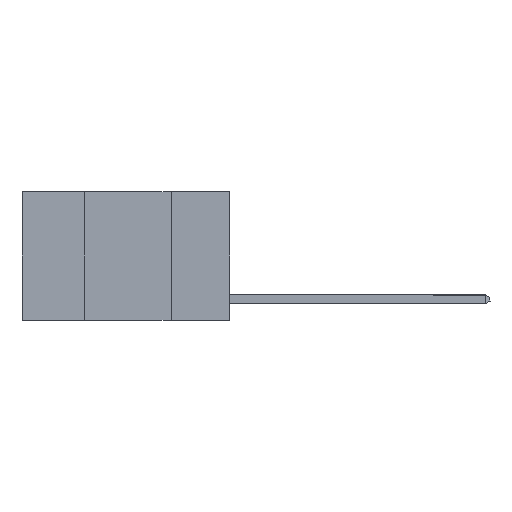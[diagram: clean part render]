
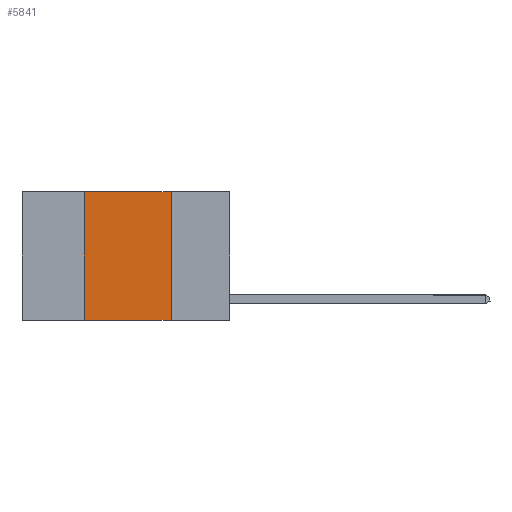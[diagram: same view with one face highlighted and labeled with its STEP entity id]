
A CAD part, left-side view. The second image highlights one B-rep face of the part: STEP entity #5841.
In plain terms, the highlighted planar face has unit normal (-1, 0, 0).
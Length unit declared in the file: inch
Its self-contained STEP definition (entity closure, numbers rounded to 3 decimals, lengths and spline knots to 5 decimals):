
#486 = LINE ( 'NONE', #6001, #4030 ) ;
#499 = EDGE_CURVE ( 'NONE', #4530, #4029, #4433, .T. ) ;
#816 = CARTESIAN_POINT ( 'NONE',  ( 0., 0.42, 0. ) ) ;
#873 = LINE ( 'NONE', #2866, #8140 ) ;
#902 = DIRECTION ( 'NONE',  ( 1., 0., 0. ) ) ;
#1607 = DIRECTION ( 'NONE',  ( 0., -1., 0. ) ) ;
#2190 = LINE ( 'NONE', #3654, #5828 ) ;
#2866 = CARTESIAN_POINT ( 'NONE',  ( 0., 0.42, 0. ) ) ;
#2947 = EDGE_CURVE ( 'NONE', #5457, #4029, #2190, .T. ) ;
#3586 = DIRECTION ( 'NONE',  ( 0., 0., 1. ) ) ;
#3654 = CARTESIAN_POINT ( 'NONE',  ( 0., 0.6, -0.37 ) ) ;
#3820 = CARTESIAN_POINT ( 'NONE',  ( 0., 0.17, 0. ) ) ;
#3882 = PLANE ( 'NONE',  #5989 ) ;
#4029 = VERTEX_POINT ( 'NONE', #6752 ) ;
#4030 = VECTOR ( 'NONE', #1607, 39.37008 ) ;
#4433 = LINE ( 'NONE', #3820, #8183 ) ;
#4530 = VERTEX_POINT ( 'NONE', #8674 ) ;
#4539 = DIRECTION ( 'NONE',  ( 0., 0., -1. ) ) ;
#4798 = CARTESIAN_POINT ( 'NONE',  ( 0., 0.42, -0.37 ) ) ;
#4890 = ORIENTED_EDGE ( 'NONE', *, *, #499, .F. ) ;
#5123 = ORIENTED_EDGE ( 'NONE', *, *, #6675, .F. ) ;
#5340 = CARTESIAN_POINT ( 'NONE',  ( 0., 0.6, 0. ) ) ;
#5457 = VERTEX_POINT ( 'NONE', #4798 ) ;
#5828 = VECTOR ( 'NONE', #7919, 39.37008 ) ;
#5841 = ADVANCED_FACE ( 'NONE', ( #7607 ), #3882, .F. ) ;
#5989 = AXIS2_PLACEMENT_3D ( 'NONE', #5340, #902, #6048 ) ;
#6001 = CARTESIAN_POINT ( 'NONE',  ( 0., 0.6, 0. ) ) ;
#6048 = DIRECTION ( 'NONE',  ( 0., 0., -1. ) ) ;
#6413 = EDGE_CURVE ( 'NONE', #5457, #8448, #873, .T. ) ;
#6675 = EDGE_CURVE ( 'NONE', #8448, #4530, #486, .T. ) ;
#6752 = CARTESIAN_POINT ( 'NONE',  ( 0., 0.17, -0.37 ) ) ;
#6988 = ORIENTED_EDGE ( 'NONE', *, *, #6413, .F. ) ;
#7607 = FACE_OUTER_BOUND ( 'NONE', #8508, .T. ) ;
#7919 = DIRECTION ( 'NONE',  ( 0., -1., 0. ) ) ;
#8140 = VECTOR ( 'NONE', #3586, 39.37008 ) ;
#8183 = VECTOR ( 'NONE', #4539, 39.37008 ) ;
#8448 = VERTEX_POINT ( 'NONE', #816 ) ;
#8508 = EDGE_LOOP ( 'NONE', ( #4890, #5123, #6988, #8848 ) ) ;
#8674 = CARTESIAN_POINT ( 'NONE',  ( 0., 0.17, 0. ) ) ;
#8848 = ORIENTED_EDGE ( 'NONE', *, *, #2947, .T. ) ;
